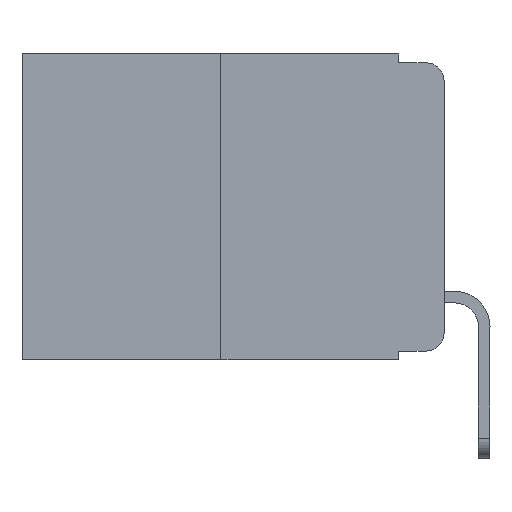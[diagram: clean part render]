
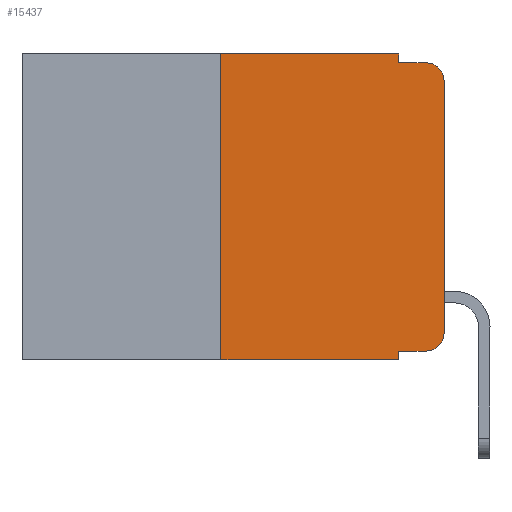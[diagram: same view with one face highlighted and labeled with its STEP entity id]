
A CAD part, left-side view. The second image highlights one B-rep face of the part: STEP entity #15437.
In plain terms, the highlighted planar face has unit normal (-1, 0, 0).
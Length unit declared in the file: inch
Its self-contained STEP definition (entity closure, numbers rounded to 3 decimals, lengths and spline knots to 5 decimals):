
#189 = CARTESIAN_POINT ( 'NONE',  ( 0., 0.02, -0.03 ) ) ;
#366 = LINE ( 'NONE', #1978, #2689 ) ;
#515 = ORIENTED_EDGE ( 'NONE', *, *, #1567, .T. ) ;
#850 = CARTESIAN_POINT ( 'NONE',  ( 0., 0.02, -0.313 ) ) ;
#1121 = DIRECTION ( 'NONE',  ( 0., -1., 0. ) ) ;
#1127 = VERTEX_POINT ( 'NONE', #12499 ) ;
#1567 = EDGE_CURVE ( 'NONE', #8587, #12724, #4252, .T. ) ;
#1617 = CARTESIAN_POINT ( 'NONE',  ( 0., 0.051, -0.333 ) ) ;
#1911 = EDGE_CURVE ( 'NONE', #5543, #6801, #13689, .T. ) ;
#1978 = CARTESIAN_POINT ( 'NONE',  ( 0., 0.473, -0.343 ) ) ;
#2011 = VECTOR ( 'NONE', #7078, 39.37008 ) ;
#2034 = AXIS2_PLACEMENT_3D ( 'NONE', #850, #4343, #14220 ) ;
#2095 = EDGE_CURVE ( 'NONE', #10005, #2941, #2107, .T. ) ;
#2107 = LINE ( 'NONE', #2529, #9861 ) ;
#2270 = EDGE_CURVE ( 'NONE', #1127, #8587, #13473, .T. ) ;
#2327 = VECTOR ( 'NONE', #8520, 39.37008 ) ;
#2375 = EDGE_CURVE ( 'NONE', #10005, #9303, #366, .T. ) ;
#2529 = CARTESIAN_POINT ( 'NONE',  ( 0., 0.25, 0. ) ) ;
#2671 = DIRECTION ( 'NONE',  ( -1., 0., 0. ) ) ;
#2689 = VECTOR ( 'NONE', #3213, 39.37008 ) ;
#2941 = VERTEX_POINT ( 'NONE', #11573 ) ;
#3213 = DIRECTION ( 'NONE',  ( 0., -1., 0. ) ) ;
#3303 = LINE ( 'NONE', #1617, #12761 ) ;
#4170 = CARTESIAN_POINT ( 'NONE',  ( 0., 0.051, 0. ) ) ;
#4252 = LINE ( 'NONE', #10869, #2327 ) ;
#4343 = DIRECTION ( 'NONE',  ( -1., 0., 0. ) ) ;
#4766 = LINE ( 'NONE', #7049, #8631 ) ;
#5409 = ORIENTED_EDGE ( 'NONE', *, *, #9832, .T. ) ;
#5511 = FACE_OUTER_BOUND ( 'NONE', #9461, .T. ) ;
#5543 = VERTEX_POINT ( 'NONE', #8543 ) ;
#5996 = DIRECTION ( 'NONE',  ( 1., 0., 0. ) ) ;
#6351 = AXIS2_PLACEMENT_3D ( 'NONE', #189, #2671, #10238 ) ;
#6801 = VERTEX_POINT ( 'NONE', #12130 ) ;
#6967 = EDGE_CURVE ( 'NONE', #10880, #5543, #4766, .T. ) ;
#7049 = CARTESIAN_POINT ( 'NONE',  ( 0., 0.051, 0. ) ) ;
#7078 = DIRECTION ( 'NONE',  ( 0., -1., 0. ) ) ;
#7795 = CARTESIAN_POINT ( 'NONE',  ( 0., 0., -0.03 ) ) ;
#7981 = EDGE_CURVE ( 'NONE', #12724, #6801, #13011, .T. ) ;
#8367 = EDGE_CURVE ( 'NONE', #2941, #10880, #9158, .T. ) ;
#8520 = DIRECTION ( 'NONE',  ( 0., 0., 1. ) ) ;
#8543 = CARTESIAN_POINT ( 'NONE',  ( 0., 0.051, -0.01 ) ) ;
#8587 = VERTEX_POINT ( 'NONE', #14804 ) ;
#8631 = VECTOR ( 'NONE', #12035, 39.37008 ) ;
#8652 = ORIENTED_EDGE ( 'NONE', *, *, #11087, .F. ) ;
#8695 = ORIENTED_EDGE ( 'NONE', *, *, #1911, .F. ) ;
#9003 = ORIENTED_EDGE ( 'NONE', *, *, #2375, .T. ) ;
#9158 = LINE ( 'NONE', #15285, #2011 ) ;
#9303 = VERTEX_POINT ( 'NONE', #11489 ) ;
#9461 = EDGE_LOOP ( 'NONE', ( #515, #12662, #8695, #9558, #10326, #11220, #9003, #8652, #5409, #15597 ) ) ;
#9558 = ORIENTED_EDGE ( 'NONE', *, *, #6967, .F. ) ;
#9653 = AXIS2_PLACEMENT_3D ( 'NONE', #10966, #5996, #14611 ) ;
#9824 = CARTESIAN_POINT ( 'NONE',  ( 0., 0.051, 0. ) ) ;
#9832 = EDGE_CURVE ( 'NONE', #11615, #1127, #3303, .T. ) ;
#9861 = VECTOR ( 'NONE', #9893, 39.37008 ) ;
#9893 = DIRECTION ( 'NONE',  ( 0., 0., 1. ) ) ;
#10005 = VERTEX_POINT ( 'NONE', #12813 ) ;
#10062 = CARTESIAN_POINT ( 'NONE',  ( 0., 0.051, -0.333 ) ) ;
#10238 = DIRECTION ( 'NONE',  ( 0., 0., -1. ) ) ;
#10247 = DIRECTION ( 'NONE',  ( 0., -1., 0. ) ) ;
#10326 = ORIENTED_EDGE ( 'NONE', *, *, #8367, .F. ) ;
#10419 = LINE ( 'NONE', #4170, #12337 ) ;
#10869 = CARTESIAN_POINT ( 'NONE',  ( 0., 0., 0. ) ) ;
#10880 = VERTEX_POINT ( 'NONE', #9824 ) ;
#10966 = CARTESIAN_POINT ( 'NONE',  ( 0., 0.473, 0. ) ) ;
#11087 = EDGE_CURVE ( 'NONE', #11615, #9303, #10419, .T. ) ;
#11220 = ORIENTED_EDGE ( 'NONE', *, *, #2095, .F. ) ;
#11489 = CARTESIAN_POINT ( 'NONE',  ( 0., 0.051, -0.343 ) ) ;
#11573 = CARTESIAN_POINT ( 'NONE',  ( 0., 0.25, 0. ) ) ;
#11615 = VERTEX_POINT ( 'NONE', #10062 ) ;
#11626 = DIRECTION ( 'NONE',  ( 0., 0., -1. ) ) ;
#11770 = VECTOR ( 'NONE', #1121, 39.37008 ) ;
#12035 = DIRECTION ( 'NONE',  ( 0., 0., -1. ) ) ;
#12111 = CARTESIAN_POINT ( 'NONE',  ( 0., 0.051, -0.01 ) ) ;
#12130 = CARTESIAN_POINT ( 'NONE',  ( 0., 0.02, -0.01 ) ) ;
#12337 = VECTOR ( 'NONE', #11626, 39.37008 ) ;
#12499 = CARTESIAN_POINT ( 'NONE',  ( 0., 0.02, -0.333 ) ) ;
#12662 = ORIENTED_EDGE ( 'NONE', *, *, #7981, .T. ) ;
#12724 = VERTEX_POINT ( 'NONE', #7795 ) ;
#12761 = VECTOR ( 'NONE', #10247, 39.37008 ) ;
#12813 = CARTESIAN_POINT ( 'NONE',  ( 0., 0.25, -0.343 ) ) ;
#13011 = CIRCLE ( 'NONE', #6351, 0.02 ) ;
#13473 = CIRCLE ( 'NONE', #2034, 0.02 ) ;
#13689 = LINE ( 'NONE', #12111, #11770 ) ;
#14220 = DIRECTION ( 'NONE',  ( 0., 0., -1. ) ) ;
#14611 = DIRECTION ( 'NONE',  ( 0., 0., -1. ) ) ;
#14720 = PLANE ( 'NONE',  #9653 ) ;
#14804 = CARTESIAN_POINT ( 'NONE',  ( 0., 0., -0.313 ) ) ;
#15285 = CARTESIAN_POINT ( 'NONE',  ( 0., 0.473, 0. ) ) ;
#15437 = ADVANCED_FACE ( 'NONE', ( #5511 ), #14720, .F. ) ;
#15597 = ORIENTED_EDGE ( 'NONE', *, *, #2270, .T. ) ;
